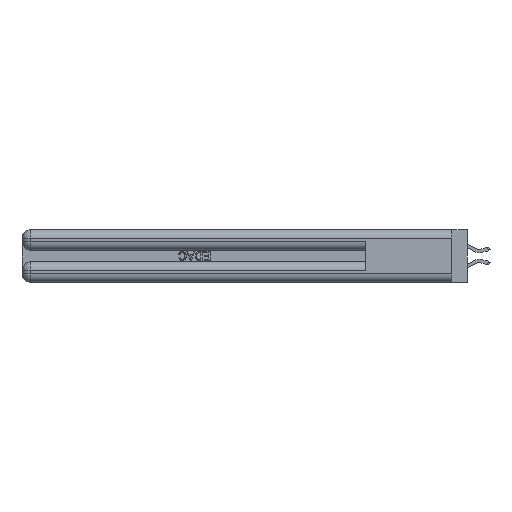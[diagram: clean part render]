
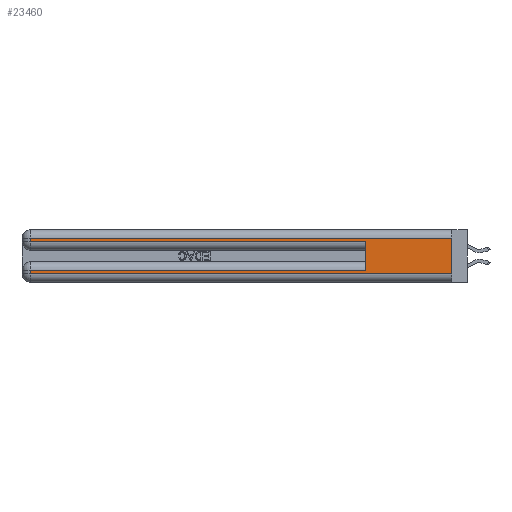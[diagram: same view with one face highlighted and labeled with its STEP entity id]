
A CAD part, left-side view. The second image highlights one B-rep face of the part: STEP entity #23460.
In plain terms, the highlighted planar face has unit normal (-1, 0, 0).
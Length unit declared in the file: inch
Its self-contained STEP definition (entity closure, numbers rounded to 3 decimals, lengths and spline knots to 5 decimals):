
#1165 = ORIENTED_EDGE ( 'NONE', *, *, #1616, .T. ) ;
#1616 = EDGE_CURVE ( 'NONE', #21293, #43867, #24599, .T. ) ;
#2197 = DIRECTION ( 'NONE',  ( 0., 0., -1. ) ) ;
#2325 = CARTESIAN_POINT ( 'NONE',  ( 0., 2.94, 0.37 ) ) ;
#3132 = DIRECTION ( 'NONE',  ( 1., 0., 0. ) ) ;
#3178 = VERTEX_POINT ( 'NONE', #12383 ) ;
#3198 = EDGE_CURVE ( 'NONE', #42824, #21293, #29038, .T. ) ;
#5551 = DIRECTION ( 'NONE',  ( 0., 0., -1. ) ) ;
#5849 = VERTEX_POINT ( 'NONE', #27302 ) ;
#6133 = VECTOR ( 'NONE', #10273, 39.37008 ) ;
#7606 = CARTESIAN_POINT ( 'NONE',  ( 0., 2.94, 0.31 ) ) ;
#7661 = EDGE_CURVE ( 'NONE', #29988, #3178, #31034, .T. ) ;
#8195 = VERTEX_POINT ( 'NONE', #7606 ) ;
#9181 = VECTOR ( 'NONE', #2197, 39.37008 ) ;
#10045 = DIRECTION ( 'NONE',  ( 0., -1., 0. ) ) ;
#10273 = DIRECTION ( 'NONE',  ( 0., -1., 0. ) ) ;
#11494 = VECTOR ( 'NONE', #10045, 39.37008 ) ;
#11650 = VECTOR ( 'NONE', #35679, 39.37008 ) ;
#12148 = ORIENTED_EDGE ( 'NONE', *, *, #7661, .F. ) ;
#12370 = CARTESIAN_POINT ( 'NONE',  ( 0., 2.94, 0.085 ) ) ;
#12383 = CARTESIAN_POINT ( 'NONE',  ( 0., 0., 0.06 ) ) ;
#15158 = EDGE_CURVE ( 'NONE', #8195, #35611, #22249, .T. ) ;
#15197 = DIRECTION ( 'NONE',  ( 0., 0., -1. ) ) ;
#15899 = VECTOR ( 'NONE', #15197, 39.37008 ) ;
#17004 = CARTESIAN_POINT ( 'NONE',  ( 0., 0.6, 0.085 ) ) ;
#17232 = CARTESIAN_POINT ( 'NONE',  ( 0., 0., 0.285 ) ) ;
#17628 = ORIENTED_EDGE ( 'NONE', *, *, #39116, .T. ) ;
#19236 = EDGE_LOOP ( 'NONE', ( #12148, #17628, #35688, #42310, #36089, #33554, #1165, #28526 ) ) ;
#20680 = CARTESIAN_POINT ( 'NONE',  ( 0., 0., 0.37 ) ) ;
#21244 = CARTESIAN_POINT ( 'NONE',  ( 0., 2.94, 0.37 ) ) ;
#21293 = VERTEX_POINT ( 'NONE', #12370 ) ;
#21313 = LINE ( 'NONE', #17232, #11494 ) ;
#21368 = CARTESIAN_POINT ( 'NONE',  ( 0., 0.6, 0.145 ) ) ;
#22179 = CARTESIAN_POINT ( 'NONE',  ( 0., 2.94, 0.285 ) ) ;
#22249 = LINE ( 'NONE', #2325, #28615 ) ;
#23460 = ADVANCED_FACE ( 'NONE', ( #36372 ), #43461, .F. ) ;
#24417 = CARTESIAN_POINT ( 'NONE',  ( 0., 0., 0.06 ) ) ;
#24599 = LINE ( 'NONE', #21244, #15899 ) ;
#27302 = CARTESIAN_POINT ( 'NONE',  ( 0., 0.6, 0.285 ) ) ;
#28526 = ORIENTED_EDGE ( 'NONE', *, *, #38086, .T. ) ;
#28615 = VECTOR ( 'NONE', #5551, 39.37008 ) ;
#29038 = LINE ( 'NONE', #47548, #31344 ) ;
#29988 = VERTEX_POINT ( 'NONE', #43299 ) ;
#30847 = LINE ( 'NONE', #24417, #6133 ) ;
#31034 = LINE ( 'NONE', #20680, #9181 ) ;
#31099 = AXIS2_PLACEMENT_3D ( 'NONE', #36541, #3132, #32988 ) ;
#31249 = LINE ( 'NONE', #21368, #11650 ) ;
#31344 = VECTOR ( 'NONE', #35389, 39.37008 ) ;
#32988 = DIRECTION ( 'NONE',  ( 0., 0., -1. ) ) ;
#33554 = ORIENTED_EDGE ( 'NONE', *, *, #3198, .T. ) ;
#33726 = CARTESIAN_POINT ( 'NONE',  ( 0., 2.94, 0.06 ) ) ;
#35389 = DIRECTION ( 'NONE',  ( 0., 1., 0. ) ) ;
#35611 = VERTEX_POINT ( 'NONE', #22179 ) ;
#35679 = DIRECTION ( 'NONE',  ( 0., 0., 1. ) ) ;
#35688 = ORIENTED_EDGE ( 'NONE', *, *, #15158, .T. ) ;
#36089 = ORIENTED_EDGE ( 'NONE', *, *, #46013, .F. ) ;
#36372 = FACE_OUTER_BOUND ( 'NONE', #19236, .T. ) ;
#36541 = CARTESIAN_POINT ( 'NONE',  ( 0., 0., 0.37 ) ) ;
#38086 = EDGE_CURVE ( 'NONE', #43867, #3178, #30847, .T. ) ;
#39116 = EDGE_CURVE ( 'NONE', #29988, #8195, #41044, .T. ) ;
#39943 = VECTOR ( 'NONE', #45715, 39.37008 ) ;
#41044 = LINE ( 'NONE', #45869, #39943 ) ;
#42052 = EDGE_CURVE ( 'NONE', #35611, #5849, #21313, .T. ) ;
#42310 = ORIENTED_EDGE ( 'NONE', *, *, #42052, .T. ) ;
#42824 = VERTEX_POINT ( 'NONE', #17004 ) ;
#43299 = CARTESIAN_POINT ( 'NONE',  ( 0., 0., 0.31 ) ) ;
#43461 = PLANE ( 'NONE',  #31099 ) ;
#43867 = VERTEX_POINT ( 'NONE', #33726 ) ;
#45715 = DIRECTION ( 'NONE',  ( 0., 1., 0. ) ) ;
#45869 = CARTESIAN_POINT ( 'NONE',  ( 0., 0., 0.31 ) ) ;
#46013 = EDGE_CURVE ( 'NONE', #42824, #5849, #31249, .T. ) ;
#47548 = CARTESIAN_POINT ( 'NONE',  ( 0., 0., 0.085 ) ) ;
